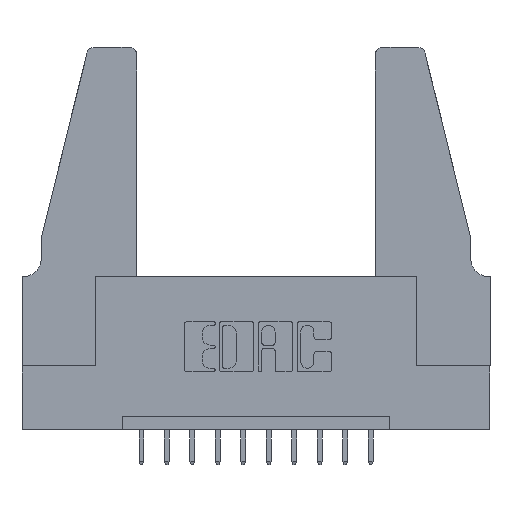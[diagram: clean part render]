
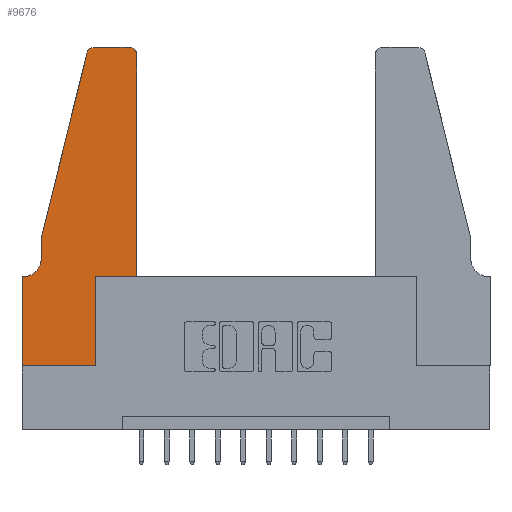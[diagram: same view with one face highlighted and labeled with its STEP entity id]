
A CAD part, top view. The second image highlights one B-rep face of the part: STEP entity #9676.
In plain terms, the highlighted planar face has unit normal (0, 0, 1).
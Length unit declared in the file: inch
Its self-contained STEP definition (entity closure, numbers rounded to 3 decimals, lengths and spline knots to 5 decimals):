
#68 = PLANE ( 'NONE',  #6090 ) ;
#366 = VECTOR ( 'NONE', #2920, 39.37008 ) ;
#542 = VECTOR ( 'NONE', #10280, 39.37008 ) ;
#771 = EDGE_CURVE ( 'NONE', #6926, #3709, #11494, .T. ) ;
#882 = VECTOR ( 'NONE', #12507, 39.37008 ) ;
#915 = CARTESIAN_POINT ( 'NONE',  ( 0., 0.35, 0.37 ) ) ;
#1243 = DIRECTION ( 'NONE',  ( -0.239, -0.971, 0. ) ) ;
#1455 = ORIENTED_EDGE ( 'NONE', *, *, #3659, .T. ) ;
#1708 = EDGE_CURVE ( 'NONE', #5105, #14084, #10204, .T. ) ;
#2057 = AXIS2_PLACEMENT_3D ( 'NONE', #10917, #7907, #6694 ) ;
#2329 = DIRECTION ( 'NONE',  ( 0., 1., 0. ) ) ;
#2342 = LINE ( 'NONE', #3418, #3104 ) ;
#2353 = DIRECTION ( 'NONE',  ( 1., 0., 0. ) ) ;
#2438 = VERTEX_POINT ( 'NONE', #6690 ) ;
#2449 = EDGE_CURVE ( 'NONE', #3709, #10986, #5554, .T. ) ;
#2546 = DIRECTION ( 'NONE',  ( -1., 0., 0. ) ) ;
#2920 = DIRECTION ( 'NONE',  ( 0., -1., 0. ) ) ;
#3104 = VECTOR ( 'NONE', #2546, 39.37008 ) ;
#3207 = CIRCLE ( 'NONE', #2057, 0.03 ) ;
#3418 = CARTESIAN_POINT ( 'NONE',  ( 0.2605, 1.25, 0.37 ) ) ;
#3431 = LINE ( 'NONE', #13075, #3916 ) ;
#3487 = DIRECTION ( 'NONE',  ( 1., 0., 0. ) ) ;
#3659 = EDGE_CURVE ( 'NONE', #10857, #12435, #7875, .T. ) ;
#3709 = VERTEX_POINT ( 'NONE', #13058 ) ;
#3789 = EDGE_CURVE ( 'NONE', #7641, #6926, #2342, .T. ) ;
#3893 = ORIENTED_EDGE ( 'NONE', *, *, #2449, .T. ) ;
#3916 = VECTOR ( 'NONE', #6778, 39.37008 ) ;
#4000 = EDGE_CURVE ( 'NONE', #10986, #10857, #4991, .T. ) ;
#4159 = EDGE_CURVE ( 'NONE', #5707, #9796, #11828, .T. ) ;
#4446 = DIRECTION ( 'NONE',  ( 0., 0., 1. ) ) ;
#4991 = LINE ( 'NONE', #11403, #366 ) ;
#5091 = CARTESIAN_POINT ( 'NONE',  ( 0., 0., 0.37 ) ) ;
#5105 = VERTEX_POINT ( 'NONE', #915 ) ;
#5344 = AXIS2_PLACEMENT_3D ( 'NONE', #11054, #4446, #2353 ) ;
#5356 = ORIENTED_EDGE ( 'NONE', *, *, #8970, .T. ) ;
#5554 = LINE ( 'NONE', #12108, #14008 ) ;
#5639 = ORIENTED_EDGE ( 'NONE', *, *, #5718, .T. ) ;
#5707 = VERTEX_POINT ( 'NONE', #9108 ) ;
#5718 = EDGE_CURVE ( 'NONE', #2438, #5707, #11096, .T. ) ;
#6090 = AXIS2_PLACEMENT_3D ( 'NONE', #6691, #10975, #3487 ) ;
#6248 = ORIENTED_EDGE ( 'NONE', *, *, #3789, .T. ) ;
#6261 = DIRECTION ( 'NONE',  ( 1., 0., 0. ) ) ;
#6326 = VECTOR ( 'NONE', #2329, 39.37008 ) ;
#6348 = CARTESIAN_POINT ( 'NONE',  ( 0.0055, 0.42, 0.37 ) ) ;
#6353 = CARTESIAN_POINT ( 'NONE',  ( 0.0755, 0.42, 0.37 ) ) ;
#6560 = DIRECTION ( 'NONE',  ( 0., 0., -1. ) ) ;
#6600 = CARTESIAN_POINT ( 'NONE',  ( 0., 0., 0.37 ) ) ;
#6690 = CARTESIAN_POINT ( 'NONE',  ( 0.2865, 0., 0.37 ) ) ;
#6691 = CARTESIAN_POINT ( 'NONE',  ( 0., 0.35, 0.37 ) ) ;
#6694 = DIRECTION ( 'NONE',  ( 1., 0., 0. ) ) ;
#6778 = DIRECTION ( 'NONE',  ( 1., 0., 0. ) ) ;
#6926 = VERTEX_POINT ( 'NONE', #10632 ) ;
#7128 = ORIENTED_EDGE ( 'NONE', *, *, #4159, .T. ) ;
#7482 = ORIENTED_EDGE ( 'NONE', *, *, #11531, .T. ) ;
#7484 = LINE ( 'NONE', #12035, #11890 ) ;
#7641 = VERTEX_POINT ( 'NONE', #12284 ) ;
#7875 = CIRCLE ( 'NONE', #11757, 0.07 ) ;
#7884 = VECTOR ( 'NONE', #6261, 39.37008 ) ;
#7907 = DIRECTION ( 'NONE',  ( 0., 0., 1. ) ) ;
#8042 = CARTESIAN_POINT ( 'NONE',  ( 0.2865, 0.35, 0.37 ) ) ;
#8299 = CARTESIAN_POINT ( 'NONE',  ( 0.4505, 1.22, 0.37 ) ) ;
#8561 = CARTESIAN_POINT ( 'NONE',  ( 0.0055, 0.35, 0.37 ) ) ;
#8970 = EDGE_CURVE ( 'NONE', #9796, #10773, #13713, .T. ) ;
#9108 = CARTESIAN_POINT ( 'NONE',  ( 0.2865, 0.35, 0.37 ) ) ;
#9118 = ORIENTED_EDGE ( 'NONE', *, *, #771, .T. ) ;
#9303 = CARTESIAN_POINT ( 'NONE',  ( 0.4505, 0.35, 0.37 ) ) ;
#9676 = ADVANCED_FACE ( 'NONE', ( #10026 ), #68, .T. ) ;
#9796 = VERTEX_POINT ( 'NONE', #11108 ) ;
#10026 = FACE_OUTER_BOUND ( 'NONE', #11833, .T. ) ;
#10204 = LINE ( 'NONE', #5091, #542 ) ;
#10280 = DIRECTION ( 'NONE',  ( 0., -1., 0. ) ) ;
#10559 = ORIENTED_EDGE ( 'NONE', *, *, #4000, .T. ) ;
#10632 = CARTESIAN_POINT ( 'NONE',  ( 0.284, 1.25, 0.37 ) ) ;
#10773 = VERTEX_POINT ( 'NONE', #8299 ) ;
#10857 = VERTEX_POINT ( 'NONE', #6353 ) ;
#10913 = DIRECTION ( 'NONE',  ( -1., 0., 0. ) ) ;
#10917 = CARTESIAN_POINT ( 'NONE',  ( 0.4205, 1.22, 0.37 ) ) ;
#10975 = DIRECTION ( 'NONE',  ( 0., 0., 1. ) ) ;
#10986 = VERTEX_POINT ( 'NONE', #12184 ) ;
#11036 = EDGE_CURVE ( 'NONE', #10773, #7641, #3207, .T. ) ;
#11054 = CARTESIAN_POINT ( 'NONE',  ( 0.284, 1.22, 0.37 ) ) ;
#11096 = LINE ( 'NONE', #8042, #6326 ) ;
#11108 = CARTESIAN_POINT ( 'NONE',  ( 0.4505, 0.35, 0.37 ) ) ;
#11403 = CARTESIAN_POINT ( 'NONE',  ( 0.0755, 0.5, 0.37 ) ) ;
#11494 = CIRCLE ( 'NONE', #5344, 0.03 ) ;
#11531 = EDGE_CURVE ( 'NONE', #14084, #2438, #3431, .T. ) ;
#11757 = AXIS2_PLACEMENT_3D ( 'NONE', #6348, #6560, #10913 ) ;
#11827 = DIRECTION ( 'NONE',  ( -1., 0., 0. ) ) ;
#11828 = LINE ( 'NONE', #14035, #7884 ) ;
#11833 = EDGE_LOOP ( 'NONE', ( #6248, #9118, #3893, #10559, #1455, #13066, #13527, #7482, #5639, #7128, #5356, #13187 ) ) ;
#11890 = VECTOR ( 'NONE', #11827, 39.37008 ) ;
#12035 = CARTESIAN_POINT ( 'NONE',  ( 0.0755, 0.35, 0.37 ) ) ;
#12108 = CARTESIAN_POINT ( 'NONE',  ( 0.0755, 0.5, 0.37 ) ) ;
#12184 = CARTESIAN_POINT ( 'NONE',  ( 0.0755, 0.5, 0.37 ) ) ;
#12284 = CARTESIAN_POINT ( 'NONE',  ( 0.4205, 1.25, 0.37 ) ) ;
#12435 = VERTEX_POINT ( 'NONE', #8561 ) ;
#12442 = EDGE_CURVE ( 'NONE', #12435, #5105, #7484, .T. ) ;
#12507 = DIRECTION ( 'NONE',  ( 0., 1., 0. ) ) ;
#13058 = CARTESIAN_POINT ( 'NONE',  ( 0.25487, 1.22718, 0.37 ) ) ;
#13066 = ORIENTED_EDGE ( 'NONE', *, *, #12442, .T. ) ;
#13075 = CARTESIAN_POINT ( 'NONE',  ( 0., 0., 0.37 ) ) ;
#13187 = ORIENTED_EDGE ( 'NONE', *, *, #11036, .T. ) ;
#13527 = ORIENTED_EDGE ( 'NONE', *, *, #1708, .T. ) ;
#13713 = LINE ( 'NONE', #9303, #882 ) ;
#14008 = VECTOR ( 'NONE', #1243, 39.37008 ) ;
#14035 = CARTESIAN_POINT ( 'NONE',  ( 0.4505, 0.35, 0.37 ) ) ;
#14084 = VERTEX_POINT ( 'NONE', #6600 ) ;
